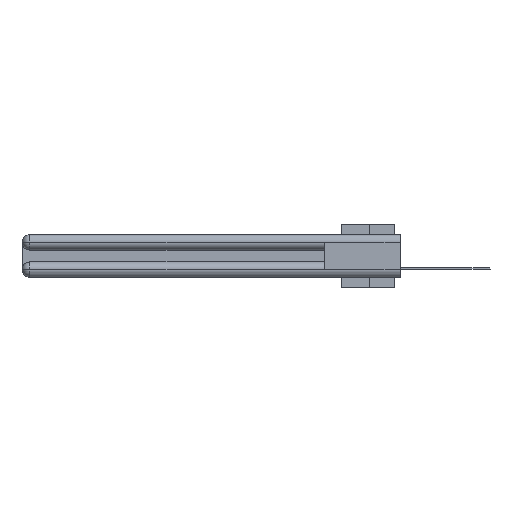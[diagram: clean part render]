
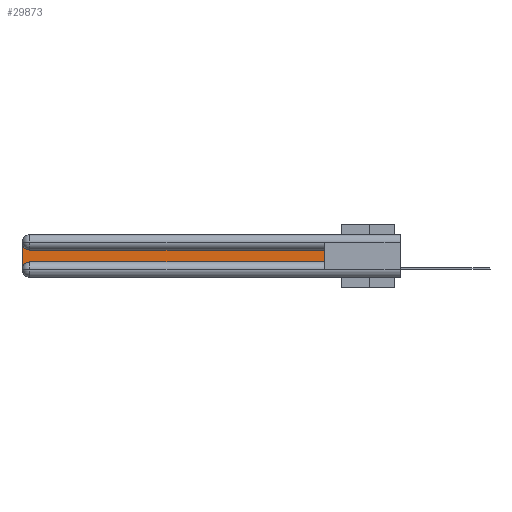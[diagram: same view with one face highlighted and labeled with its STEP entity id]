
A CAD part, left-side view. The second image highlights one B-rep face of the part: STEP entity #29873.
In plain terms, the highlighted planar face has unit normal (-1, 0, 0).
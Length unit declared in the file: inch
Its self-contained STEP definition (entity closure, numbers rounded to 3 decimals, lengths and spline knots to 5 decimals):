
#29 = EDGE_CURVE ( 'NONE', #17816, #10547, #23570, .T. ) ;
#230 = ORIENTED_EDGE ( 'NONE', *, *, #19995, .T. ) ;
#770 = DIRECTION ( 'NONE',  ( 0., 0., 1. ) ) ;
#1127 = CARTESIAN_POINT ( 'NONE',  ( 0.075, 0.6, -0.1225 ) ) ;
#1446 = CARTESIAN_POINT ( 'NONE',  ( 0.075, 2.94, -0.1225 ) ) ;
#1668 = DIRECTION ( 'NONE',  ( 0., -1., 0. ) ) ;
#2408 = AXIS2_PLACEMENT_3D ( 'NONE', #24243, #13472, #31976 ) ;
#2471 = DIRECTION ( 'NONE',  ( 0., 0., -1. ) ) ;
#2473 = VECTOR ( 'NONE', #1668, 39.37008 ) ;
#2569 = VECTOR ( 'NONE', #25118, 39.37008 ) ;
#2681 = PLANE ( 'NONE',  #13360 ) ;
#3391 = LINE ( 'NONE', #27545, #2569 ) ;
#4041 = CIRCLE ( 'NONE', #2408, 0.06 ) ;
#4994 = DIRECTION ( 'NONE',  ( 1., 0., 0. ) ) ;
#6039 = VECTOR ( 'NONE', #770, 39.37008 ) ;
#7735 = ORIENTED_EDGE ( 'NONE', *, *, #17027, .T. ) ;
#9596 = VERTEX_POINT ( 'NONE', #14769 ) ;
#10547 = VERTEX_POINT ( 'NONE', #15015 ) ;
#11004 = LINE ( 'NONE', #1127, #31298 ) ;
#12778 = CARTESIAN_POINT ( 'NONE',  ( 0.075, 2.94, -0.2175 ) ) ;
#13074 = LINE ( 'NONE', #23970, #6039 ) ;
#13360 = AXIS2_PLACEMENT_3D ( 'NONE', #26382, #23517, #2471 ) ;
#13472 = DIRECTION ( 'NONE',  ( 1., 0., 0. ) ) ;
#14769 = CARTESIAN_POINT ( 'NONE',  ( 0.075, 3., -0.0625 ) ) ;
#14908 = FACE_OUTER_BOUND ( 'NONE', #16898, .T. ) ;
#14924 = ORIENTED_EDGE ( 'NONE', *, *, #31416, .T. ) ;
#15015 = CARTESIAN_POINT ( 'NONE',  ( 0.075, 0.6, -0.2175 ) ) ;
#15459 = ORIENTED_EDGE ( 'NONE', *, *, #29, .T. ) ;
#15486 = DIRECTION ( 'NONE',  ( 0., 0., -1. ) ) ;
#15675 = CIRCLE ( 'NONE', #31531, 0.06 ) ;
#16247 = EDGE_CURVE ( 'NONE', #28443, #33749, #11004, .T. ) ;
#16898 = EDGE_LOOP ( 'NONE', ( #23859, #27508, #7735, #14924, #15459, #230 ) ) ;
#17027 = EDGE_CURVE ( 'NONE', #9596, #27770, #3391, .T. ) ;
#17567 = EDGE_CURVE ( 'NONE', #33749, #9596, #15675, .T. ) ;
#17816 = VERTEX_POINT ( 'NONE', #12778 ) ;
#19995 = EDGE_CURVE ( 'NONE', #10547, #28443, #13074, .T. ) ;
#22362 = CARTESIAN_POINT ( 'NONE',  ( 0.075, 0.6, -0.1225 ) ) ;
#22370 = DIRECTION ( 'NONE',  ( 0., 1., 0. ) ) ;
#23517 = DIRECTION ( 'NONE',  ( 1., 0., 0. ) ) ;
#23570 = LINE ( 'NONE', #32829, #2473 ) ;
#23859 = ORIENTED_EDGE ( 'NONE', *, *, #16247, .T. ) ;
#23970 = CARTESIAN_POINT ( 'NONE',  ( 0.075, 0.6, -0.2175 ) ) ;
#24243 = CARTESIAN_POINT ( 'NONE',  ( 0.075, 2.94, -0.2775 ) ) ;
#25118 = DIRECTION ( 'NONE',  ( 0., 0., -1. ) ) ;
#26382 = CARTESIAN_POINT ( 'NONE',  ( 0.075, 3., -0.1225 ) ) ;
#26565 = CARTESIAN_POINT ( 'NONE',  ( 0.075, 2.94, -0.0625 ) ) ;
#27508 = ORIENTED_EDGE ( 'NONE', *, *, #17567, .T. ) ;
#27545 = CARTESIAN_POINT ( 'NONE',  ( 0.075, 3., -0.2175 ) ) ;
#27770 = VERTEX_POINT ( 'NONE', #32563 ) ;
#28443 = VERTEX_POINT ( 'NONE', #22362 ) ;
#29873 = ADVANCED_FACE ( 'NONE', ( #14908 ), #2681, .F. ) ;
#31298 = VECTOR ( 'NONE', #22370, 39.37008 ) ;
#31416 = EDGE_CURVE ( 'NONE', #27770, #17816, #4041, .T. ) ;
#31531 = AXIS2_PLACEMENT_3D ( 'NONE', #26565, #4994, #15486 ) ;
#31976 = DIRECTION ( 'NONE',  ( 0., 0., -1. ) ) ;
#32563 = CARTESIAN_POINT ( 'NONE',  ( 0.075, 3., -0.2775 ) ) ;
#32829 = CARTESIAN_POINT ( 'NONE',  ( 0.075, 0.6, -0.2175 ) ) ;
#33749 = VERTEX_POINT ( 'NONE', #1446 ) ;
